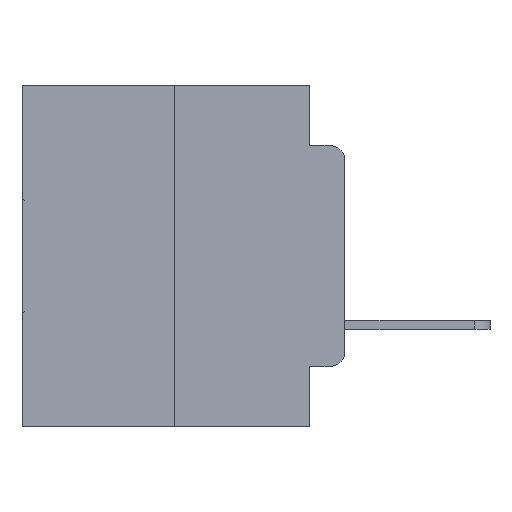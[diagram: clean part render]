
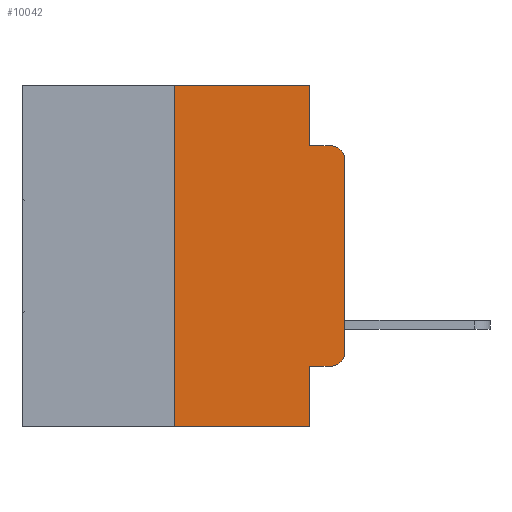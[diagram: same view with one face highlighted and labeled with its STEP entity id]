
A CAD part, left-side view. The second image highlights one B-rep face of the part: STEP entity #10042.
In plain terms, the highlighted planar face has unit normal (-1, 0, 0).
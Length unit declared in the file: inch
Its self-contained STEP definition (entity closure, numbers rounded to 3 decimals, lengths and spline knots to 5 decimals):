
#4 = DIRECTION ( 'NONE',  ( 0., -1., 0. ) ) ;
#105 = EDGE_CURVE ( 'NONE', #20950, #1159, #14376, .T. ) ;
#1159 = VERTEX_POINT ( 'NONE', #28351 ) ;
#1245 = DIRECTION ( 'NONE',  ( 0., 0., -1. ) ) ;
#1671 = DIRECTION ( 'NONE',  ( -1., 0., 0. ) ) ;
#2319 = CARTESIAN_POINT ( 'NONE',  ( 0., 0.051, -0.4115 ) ) ;
#3163 = CARTESIAN_POINT ( 'NONE',  ( 0., 0.051, 0. ) ) ;
#3282 = DIRECTION ( 'NONE',  ( 0., 0., -1. ) ) ;
#3827 = ORIENTED_EDGE ( 'NONE', *, *, #14894, .T. ) ;
#3867 = ORIENTED_EDGE ( 'NONE', *, *, #6742, .F. ) ;
#4247 = CARTESIAN_POINT ( 'NONE',  ( 0., 0.473, 0. ) ) ;
#4471 = CIRCLE ( 'NONE', #27871, 0.02 ) ;
#4676 = DIRECTION ( 'NONE',  ( 0., -1., 0. ) ) ;
#4993 = DIRECTION ( 'NONE',  ( 0., -1., 0. ) ) ;
#5190 = VERTEX_POINT ( 'NONE', #10581 ) ;
#5315 = CARTESIAN_POINT ( 'NONE',  ( 0., 0., -0.1085 ) ) ;
#5370 = CARTESIAN_POINT ( 'NONE',  ( 0., 0.02, -0.0885 ) ) ;
#6304 = VECTOR ( 'NONE', #28250, 39.37008 ) ;
#6742 = EDGE_CURVE ( 'NONE', #25527, #12830, #10093, .T. ) ;
#7581 = DIRECTION ( 'NONE',  ( 0., -1., 0. ) ) ;
#8683 = CARTESIAN_POINT ( 'NONE',  ( 0., 0.051, 0. ) ) ;
#9078 = CARTESIAN_POINT ( 'NONE',  ( 0., 0.25, 0. ) ) ;
#9150 = ORIENTED_EDGE ( 'NONE', *, *, #17137, .F. ) ;
#9379 = AXIS2_PLACEMENT_3D ( 'NONE', #25230, #16429, #1245 ) ;
#10015 = CARTESIAN_POINT ( 'NONE',  ( 0., 0.051, 0. ) ) ;
#10042 = ADVANCED_FACE ( 'NONE', ( #13067 ), #14049, .F. ) ;
#10093 = LINE ( 'NONE', #4247, #16613 ) ;
#10559 = VERTEX_POINT ( 'NONE', #11953 ) ;
#10581 = CARTESIAN_POINT ( 'NONE',  ( 0., 0., -0.3915 ) ) ;
#11102 = EDGE_LOOP ( 'NONE', ( #3827, #18601, #17536, #9150, #3867, #19319, #23096, #19702, #28580, #12529 ) ) ;
#11430 = AXIS2_PLACEMENT_3D ( 'NONE', #14505, #29798, #16849 ) ;
#11953 = CARTESIAN_POINT ( 'NONE',  ( 0., 0.02, -0.4115 ) ) ;
#12529 = ORIENTED_EDGE ( 'NONE', *, *, #20168, .T. ) ;
#12830 = VERTEX_POINT ( 'NONE', #8683 ) ;
#12843 = DIRECTION ( 'NONE',  ( 0., 0., 1. ) ) ;
#12953 = CIRCLE ( 'NONE', #11430, 0.02 ) ;
#13067 = FACE_OUTER_BOUND ( 'NONE', #11102, .T. ) ;
#13222 = CARTESIAN_POINT ( 'NONE',  ( 0., 0.25, 0. ) ) ;
#14049 = PLANE ( 'NONE',  #9379 ) ;
#14376 = LINE ( 'NONE', #23244, #29782 ) ;
#14505 = CARTESIAN_POINT ( 'NONE',  ( 0., 0.02, -0.3915 ) ) ;
#14894 = EDGE_CURVE ( 'NONE', #5190, #21918, #25643, .T. ) ;
#14948 = VECTOR ( 'NONE', #3282, 39.37008 ) ;
#15362 = LINE ( 'NONE', #13222, #20662 ) ;
#15629 = DIRECTION ( 'NONE',  ( 0., 0., 1. ) ) ;
#15707 = LINE ( 'NONE', #3163, #14948 ) ;
#16086 = EDGE_CURVE ( 'NONE', #21918, #23241, #4471, .T. ) ;
#16351 = EDGE_CURVE ( 'NONE', #19939, #23241, #18051, .T. ) ;
#16429 = DIRECTION ( 'NONE',  ( 1., 0., 0. ) ) ;
#16613 = VECTOR ( 'NONE', #4676, 39.37008 ) ;
#16768 = CARTESIAN_POINT ( 'NONE',  ( 0., 0.051, -0.4115 ) ) ;
#16799 = CARTESIAN_POINT ( 'NONE',  ( 0., 0.02, -0.1085 ) ) ;
#16849 = DIRECTION ( 'NONE',  ( 0., 0., -1. ) ) ;
#17137 = EDGE_CURVE ( 'NONE', #12830, #19939, #25113, .T. ) ;
#17311 = EDGE_CURVE ( 'NONE', #20950, #25527, #15362, .T. ) ;
#17536 = ORIENTED_EDGE ( 'NONE', *, *, #16351, .F. ) ;
#18051 = LINE ( 'NONE', #30176, #28904 ) ;
#18181 = EDGE_CURVE ( 'NONE', #24326, #1159, #15707, .T. ) ;
#18601 = ORIENTED_EDGE ( 'NONE', *, *, #16086, .T. ) ;
#18709 = EDGE_CURVE ( 'NONE', #24326, #10559, #27402, .T. ) ;
#19083 = DIRECTION ( 'NONE',  ( 0., 0., -1. ) ) ;
#19156 = VECTOR ( 'NONE', #12843, 39.37008 ) ;
#19319 = ORIENTED_EDGE ( 'NONE', *, *, #17311, .F. ) ;
#19702 = ORIENTED_EDGE ( 'NONE', *, *, #18181, .F. ) ;
#19835 = CARTESIAN_POINT ( 'NONE',  ( 0., 0., 0. ) ) ;
#19939 = VERTEX_POINT ( 'NONE', #25094 ) ;
#20168 = EDGE_CURVE ( 'NONE', #10559, #5190, #12953, .T. ) ;
#20662 = VECTOR ( 'NONE', #15629, 39.37008 ) ;
#20943 = VECTOR ( 'NONE', #4993, 39.37008 ) ;
#20950 = VERTEX_POINT ( 'NONE', #30041 ) ;
#21918 = VERTEX_POINT ( 'NONE', #5315 ) ;
#23096 = ORIENTED_EDGE ( 'NONE', *, *, #105, .T. ) ;
#23241 = VERTEX_POINT ( 'NONE', #5370 ) ;
#23244 = CARTESIAN_POINT ( 'NONE',  ( 0., 0.473, -0.5 ) ) ;
#24326 = VERTEX_POINT ( 'NONE', #16768 ) ;
#25094 = CARTESIAN_POINT ( 'NONE',  ( 0., 0.051, -0.0885 ) ) ;
#25113 = LINE ( 'NONE', #10015, #6304 ) ;
#25230 = CARTESIAN_POINT ( 'NONE',  ( 0., 0.473, 0. ) ) ;
#25527 = VERTEX_POINT ( 'NONE', #9078 ) ;
#25643 = LINE ( 'NONE', #19835, #19156 ) ;
#27402 = LINE ( 'NONE', #2319, #20943 ) ;
#27871 = AXIS2_PLACEMENT_3D ( 'NONE', #16799, #1671, #19083 ) ;
#28250 = DIRECTION ( 'NONE',  ( 0., 0., -1. ) ) ;
#28351 = CARTESIAN_POINT ( 'NONE',  ( 0., 0.051, -0.5 ) ) ;
#28580 = ORIENTED_EDGE ( 'NONE', *, *, #18709, .T. ) ;
#28904 = VECTOR ( 'NONE', #7581, 39.37008 ) ;
#29782 = VECTOR ( 'NONE', #4, 39.37008 ) ;
#29798 = DIRECTION ( 'NONE',  ( -1., 0., 0. ) ) ;
#30041 = CARTESIAN_POINT ( 'NONE',  ( 0., 0.25, -0.5 ) ) ;
#30176 = CARTESIAN_POINT ( 'NONE',  ( 0., 0.051, -0.0885 ) ) ;
